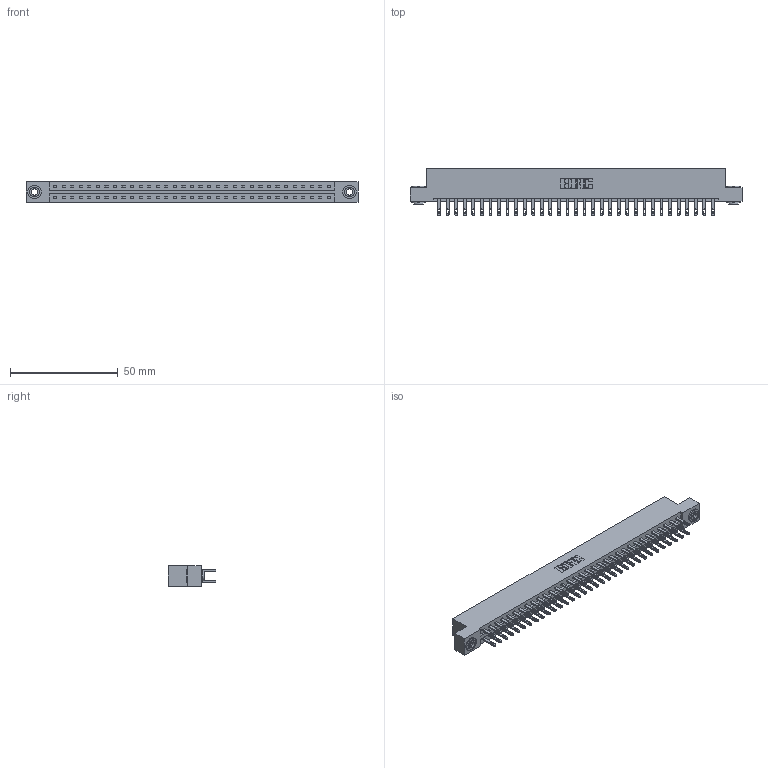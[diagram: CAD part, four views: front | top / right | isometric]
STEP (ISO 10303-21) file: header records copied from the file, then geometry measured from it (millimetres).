
FILE_DESCRIPTION (( 'STEP AP203' ), '1' );
FILE_NAME ('337-066-500-203.STEP', '2019-10-09T22:47:51', ( '' ), ( '' ), 'SwSTEP 2.0', 'SolidWorks 2016', '' );
FILE_SCHEMA (( 'CONFIG_CONTROL_DESIGN' ));
Length unit declared in the file: inch
Products named in the file (4): 337-066-500-203; 345-292-001_345-293-100; 345-250-002_345-250-002-102; 337 Part_Flush Mounting Lugs - 0.156 Dia-TH
Assembly tree (69 placements, depth 2):
  337-066-500-203
    337 Part_Flush Mounting Lugs - 0.156 Dia-TH
    345-292-001_345-293-100  x66
    345-250-002_345-250-002-102  x2
Bounding box: 153.77 x 21.85 x 9.4 mm (x, y, z)
Volume: 16306.9 mm3; surface area: 19304.3 mm2
Topology: 69 solids, 69 shells, 3452 faces, 10485 edges, 6986 vertices
Faces by surface type: plane 2192, cylinder 1252, cone 8
Entity records: 27330 total; most frequent: CARTESIAN_POINT 4585, ORIENTED_EDGE 4514, DIRECTION 3951, EDGE_CURVE 2257, VECTOR 2101, LINE 2101, VERTEX_POINT 1502, AXIS2_PLACEMENT_3D 925
